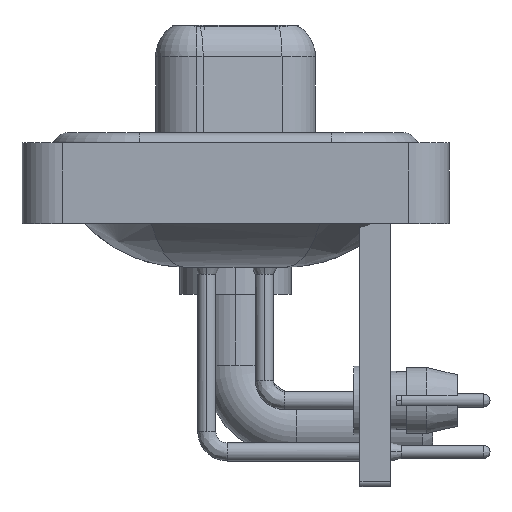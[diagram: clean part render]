
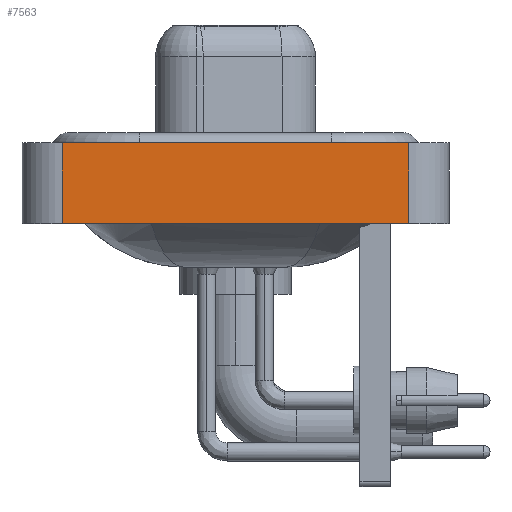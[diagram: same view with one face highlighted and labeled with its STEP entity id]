
A CAD part, left-side view. The second image highlights one B-rep face of the part: STEP entity #7563.
In plain terms, the highlighted planar face has unit normal (-1, 0, 0).
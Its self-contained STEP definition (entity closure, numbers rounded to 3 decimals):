
#497 = VERTEX_POINT ( 'NONE', #8590 ) ;
#836 = DIRECTION ( 'NONE',  ( 0., -1., 0. ) ) ;
#962 = CARTESIAN_POINT ( 'NONE',  ( -7.3, -8.55, -3.6 ) ) ;
#1278 = VECTOR ( 'NONE', #18324, 1000. ) ;
#1692 = ORIENTED_EDGE ( 'NONE', *, *, #11037, .F. ) ;
#3085 = LINE ( 'NONE', #962, #17889 ) ;
#3366 = LINE ( 'NONE', #15062, #4388 ) ;
#4388 = VECTOR ( 'NONE', #20344, 1000. ) ;
#4649 = EDGE_CURVE ( 'NONE', #7567, #497, #3366, .T. ) ;
#4871 = CARTESIAN_POINT ( 'NONE',  ( -7.3, -8.55, -3.6 ) ) ;
#5114 = PLANE ( 'NONE',  #8422 ) ;
#5424 = EDGE_LOOP ( 'NONE', ( #22188, #1692, #24543, #17195 ) ) ;
#6881 = CARTESIAN_POINT ( 'NONE',  ( -7.3, 8.55, -3.6 ) ) ;
#7563 = ADVANCED_FACE ( 'NONE', ( #15746 ), #5114, .T. ) ;
#7567 = VERTEX_POINT ( 'NONE', #6881 ) ;
#8422 = AXIS2_PLACEMENT_3D ( 'NONE', #17757, #12073, #14676 ) ;
#8590 = CARTESIAN_POINT ( 'NONE',  ( -7.3, 8.55, 0.4 ) ) ;
#10160 = CARTESIAN_POINT ( 'NONE',  ( -7.3, -8.55, -3.6 ) ) ;
#10924 = VECTOR ( 'NONE', #14219, 1000. ) ;
#11037 = EDGE_CURVE ( 'NONE', #497, #24416, #24147, .T. ) ;
#12073 = DIRECTION ( 'NONE',  ( -1., 0., 0. ) ) ;
#13653 = CARTESIAN_POINT ( 'NONE',  ( -7.3, -8.55, 0.4 ) ) ;
#14219 = DIRECTION ( 'NONE',  ( 0., -1., 0. ) ) ;
#14461 = CARTESIAN_POINT ( 'NONE',  ( -7.3, -8.55, 0.4 ) ) ;
#14676 = DIRECTION ( 'NONE',  ( 0., 0., 1. ) ) ;
#15062 = CARTESIAN_POINT ( 'NONE',  ( -7.3, 8.55, -3.6 ) ) ;
#15746 = FACE_OUTER_BOUND ( 'NONE', #5424, .T. ) ;
#15835 = LINE ( 'NONE', #10160, #1278 ) ;
#16192 = EDGE_CURVE ( 'NONE', #17215, #24416, #15835, .T. ) ;
#17195 = ORIENTED_EDGE ( 'NONE', *, *, #20826, .T. ) ;
#17215 = VERTEX_POINT ( 'NONE', #4871 ) ;
#17757 = CARTESIAN_POINT ( 'NONE',  ( -7.3, -8.55, -3.6 ) ) ;
#17889 = VECTOR ( 'NONE', #836, 1000. ) ;
#18324 = DIRECTION ( 'NONE',  ( 0., 0., 1. ) ) ;
#20344 = DIRECTION ( 'NONE',  ( 0., 0., 1. ) ) ;
#20826 = EDGE_CURVE ( 'NONE', #7567, #17215, #3085, .T. ) ;
#22188 = ORIENTED_EDGE ( 'NONE', *, *, #16192, .T. ) ;
#24147 = LINE ( 'NONE', #14461, #10924 ) ;
#24416 = VERTEX_POINT ( 'NONE', #13653 ) ;
#24543 = ORIENTED_EDGE ( 'NONE', *, *, #4649, .F. ) ;
